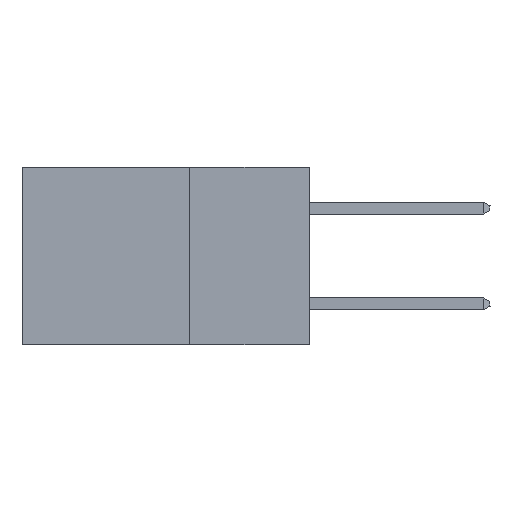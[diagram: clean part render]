
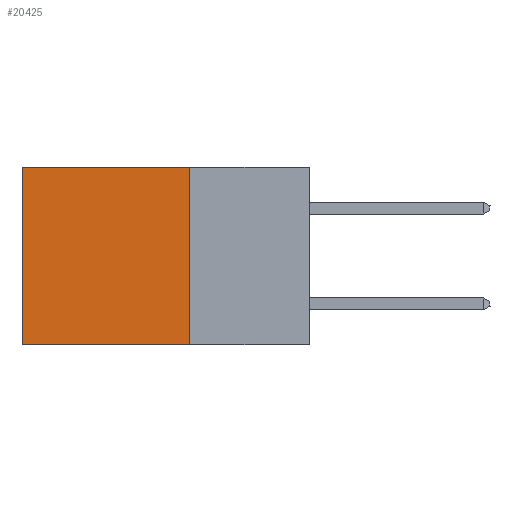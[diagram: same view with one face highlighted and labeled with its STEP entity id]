
A CAD part, left-side view. The second image highlights one B-rep face of the part: STEP entity #20425.
In plain terms, the highlighted planar face has unit normal (-1, 0, 0).
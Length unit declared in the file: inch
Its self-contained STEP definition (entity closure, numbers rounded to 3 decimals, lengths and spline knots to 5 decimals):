
#1046 = LINE ( 'NONE', #13964, #22700 ) ;
#1465 = CARTESIAN_POINT ( 'NONE',  ( 0.2875, 0.25, 0. ) ) ;
#3479 = VERTEX_POINT ( 'NONE', #28381 ) ;
#4717 = VECTOR ( 'NONE', #14980, 39.37008 ) ;
#5210 = DIRECTION ( 'NONE',  ( 0., 1., 0. ) ) ;
#5585 = CARTESIAN_POINT ( 'NONE',  ( 0.2875, 0.25, -0.37 ) ) ;
#7137 = PLANE ( 'NONE',  #24794 ) ;
#8523 = DIRECTION ( 'NONE',  ( 0., 0., -1. ) ) ;
#8908 = LINE ( 'NONE', #5585, #4717 ) ;
#10881 = CARTESIAN_POINT ( 'NONE',  ( 0.2875, 0.6, 0. ) ) ;
#13964 = CARTESIAN_POINT ( 'NONE',  ( 0.2875, 0.25, 0. ) ) ;
#14659 = CARTESIAN_POINT ( 'NONE',  ( 0.2875, 0.25, 0. ) ) ;
#14980 = DIRECTION ( 'NONE',  ( 0., 1., 0. ) ) ;
#15249 = LINE ( 'NONE', #14659, #18114 ) ;
#15332 = VERTEX_POINT ( 'NONE', #17832 ) ;
#16752 = VERTEX_POINT ( 'NONE', #33701 ) ;
#17145 = VERTEX_POINT ( 'NONE', #38476 ) ;
#17815 = EDGE_CURVE ( 'NONE', #15332, #17145, #8908, .T. ) ;
#17832 = CARTESIAN_POINT ( 'NONE',  ( 0.2875, 0.25, -0.37 ) ) ;
#18114 = VECTOR ( 'NONE', #8523, 39.37008 ) ;
#20054 = EDGE_CURVE ( 'NONE', #16752, #15332, #15249, .T. ) ;
#20409 = ORIENTED_EDGE ( 'NONE', *, *, #35932, .T. ) ;
#20425 = ADVANCED_FACE ( 'NONE', ( #32599 ), #7137, .F. ) ;
#22700 = VECTOR ( 'NONE', #5210, 39.37008 ) ;
#23688 = EDGE_CURVE ( 'NONE', #3479, #17145, #36782, .T. ) ;
#24005 = EDGE_LOOP ( 'NONE', ( #25881, #37754, #27134, #20409 ) ) ;
#24794 = AXIS2_PLACEMENT_3D ( 'NONE', #1465, #34509, #31475 ) ;
#25881 = ORIENTED_EDGE ( 'NONE', *, *, #23688, .T. ) ;
#27134 = ORIENTED_EDGE ( 'NONE', *, *, #20054, .F. ) ;
#28381 = CARTESIAN_POINT ( 'NONE',  ( 0.2875, 0.6, 0. ) ) ;
#31475 = DIRECTION ( 'NONE',  ( 0., 0., -1. ) ) ;
#31870 = DIRECTION ( 'NONE',  ( 0., 0., -1. ) ) ;
#32599 = FACE_OUTER_BOUND ( 'NONE', #24005, .T. ) ;
#33701 = CARTESIAN_POINT ( 'NONE',  ( 0.2875, 0.25, 0. ) ) ;
#34459 = VECTOR ( 'NONE', #31870, 39.37008 ) ;
#34509 = DIRECTION ( 'NONE',  ( 1., 0., 0. ) ) ;
#35932 = EDGE_CURVE ( 'NONE', #16752, #3479, #1046, .T. ) ;
#36782 = LINE ( 'NONE', #10881, #34459 ) ;
#37754 = ORIENTED_EDGE ( 'NONE', *, *, #17815, .F. ) ;
#38476 = CARTESIAN_POINT ( 'NONE',  ( 0.2875, 0.6, -0.37 ) ) ;
